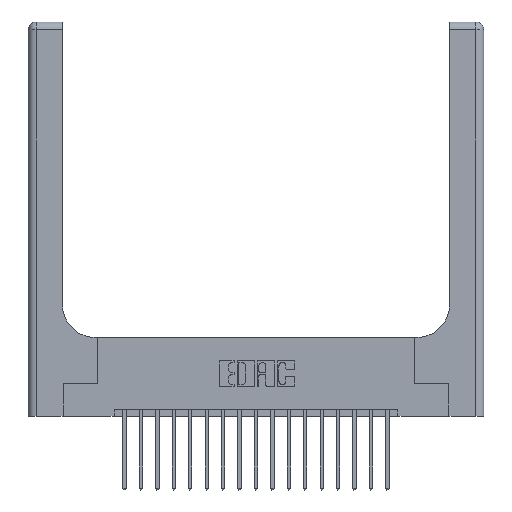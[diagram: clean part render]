
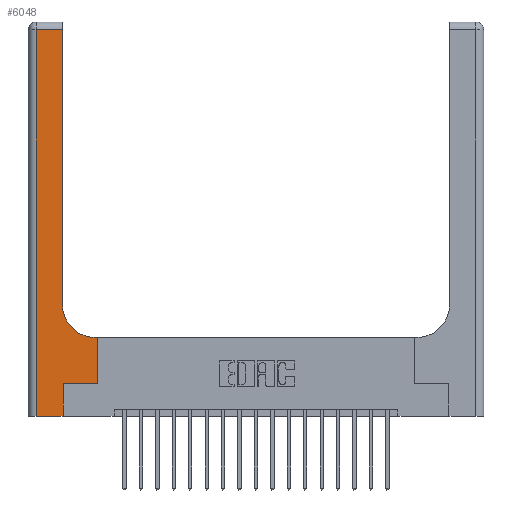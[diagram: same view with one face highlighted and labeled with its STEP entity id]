
A CAD part, top view. The second image highlights one B-rep face of the part: STEP entity #6048.
In plain terms, the highlighted planar face has unit normal (0, 0, 1).
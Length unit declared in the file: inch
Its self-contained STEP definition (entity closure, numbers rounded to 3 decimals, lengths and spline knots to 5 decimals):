
#68 = VERTEX_POINT ( 'NONE', #19939 ) ;
#161 = VERTEX_POINT ( 'NONE', #7725 ) ;
#376 = DIRECTION ( 'NONE',  ( 0., 1., 0. ) ) ;
#683 = CARTESIAN_POINT ( 'NONE',  ( 0.265, 0., 0.37 ) ) ;
#1964 = VERTEX_POINT ( 'NONE', #2599 ) ;
#2024 = CARTESIAN_POINT ( 'NONE',  ( 0.26, 3., 0.37 ) ) ;
#2301 = CARTESIAN_POINT ( 'NONE',  ( 0.26, 0.6, 0.37 ) ) ;
#2599 = CARTESIAN_POINT ( 'NONE',  ( 0.265, 0.25, 0.37 ) ) ;
#2741 = ORIENTED_EDGE ( 'NONE', *, *, #14358, .T. ) ;
#3065 = VECTOR ( 'NONE', #376, 39.37008 ) ;
#3372 = CARTESIAN_POINT ( 'NONE',  ( 0.528, 0.25, 0.37 ) ) ;
#3415 = ORIENTED_EDGE ( 'NONE', *, *, #6404, .T. ) ;
#3646 = VECTOR ( 'NONE', #11444, 39.37008 ) ;
#3700 = DIRECTION ( 'NONE',  ( -1., 0., 0. ) ) ;
#3851 = CARTESIAN_POINT ( 'NONE',  ( 0.06, 3., 0.37 ) ) ;
#3950 = EDGE_CURVE ( 'NONE', #161, #14407, #9134, .T. ) ;
#4714 = EDGE_CURVE ( 'NONE', #15654, #68, #10905, .T. ) ;
#5077 = CARTESIAN_POINT ( 'NONE',  ( 0.528, 0.6, 0.37 ) ) ;
#5481 = ORIENTED_EDGE ( 'NONE', *, *, #16665, .T. ) ;
#5692 = VECTOR ( 'NONE', #7218, 39.37008 ) ;
#5764 = CARTESIAN_POINT ( 'NONE',  ( 0.51, 0.6, 0.37 ) ) ;
#5908 = VECTOR ( 'NONE', #16442, 39.37008 ) ;
#6048 = ADVANCED_FACE ( 'NONE', ( #12311 ), #9370, .F. ) ;
#6404 = EDGE_CURVE ( 'NONE', #18203, #13740, #6736, .T. ) ;
#6592 = LINE ( 'NONE', #2024, #3065 ) ;
#6636 = VERTEX_POINT ( 'NONE', #3372 ) ;
#6736 = LINE ( 'NONE', #12910, #15665 ) ;
#7095 = DIRECTION ( 'NONE',  ( 0., -1., 0. ) ) ;
#7218 = DIRECTION ( 'NONE',  ( 1., 0., 0. ) ) ;
#7239 = ORIENTED_EDGE ( 'NONE', *, *, #19558, .T. ) ;
#7725 = CARTESIAN_POINT ( 'NONE',  ( 0.06, 0., 0.37 ) ) ;
#7795 = EDGE_CURVE ( 'NONE', #10667, #15654, #19387, .T. ) ;
#8059 = AXIS2_PLACEMENT_3D ( 'NONE', #18850, #13858, #12709 ) ;
#8204 = CARTESIAN_POINT ( 'NONE',  ( 0.26, 2.94, 0.37 ) ) ;
#8319 = LINE ( 'NONE', #17468, #3646 ) ;
#8814 = LINE ( 'NONE', #3851, #13497 ) ;
#9134 = LINE ( 'NONE', #19725, #5692 ) ;
#9370 = PLANE ( 'NONE',  #8059 ) ;
#9966 = DIRECTION ( 'NONE',  ( 1., 0., 0. ) ) ;
#10273 = DIRECTION ( 'NONE',  ( 0., 0., -1. ) ) ;
#10667 = VERTEX_POINT ( 'NONE', #5077 ) ;
#10905 = CIRCLE ( 'NONE', #15479, 0.25 ) ;
#11444 = DIRECTION ( 'NONE',  ( 0., 1., 0. ) ) ;
#11721 = VECTOR ( 'NONE', #14621, 39.37008 ) ;
#12311 = FACE_OUTER_BOUND ( 'NONE', #15535, .T. ) ;
#12709 = DIRECTION ( 'NONE',  ( -1., 0., 0. ) ) ;
#12910 = CARTESIAN_POINT ( 'NONE',  ( 0., 2.94, 0.37 ) ) ;
#13008 = ORIENTED_EDGE ( 'NONE', *, *, #3950, .T. ) ;
#13131 = DIRECTION ( 'NONE',  ( -1., 0., 0. ) ) ;
#13302 = CARTESIAN_POINT ( 'NONE',  ( 0.51, 0.85, 0.37 ) ) ;
#13497 = VECTOR ( 'NONE', #7095, 39.37008 ) ;
#13690 = CARTESIAN_POINT ( 'NONE',  ( 0.265, 0.25, 0.37 ) ) ;
#13740 = VERTEX_POINT ( 'NONE', #14294 ) ;
#13858 = DIRECTION ( 'NONE',  ( 0., 0., -1. ) ) ;
#14294 = CARTESIAN_POINT ( 'NONE',  ( 0.06, 2.94, 0.37 ) ) ;
#14358 = EDGE_CURVE ( 'NONE', #14407, #1964, #19202, .T. ) ;
#14363 = EDGE_CURVE ( 'NONE', #6636, #10667, #8319, .T. ) ;
#14407 = VERTEX_POINT ( 'NONE', #17572 ) ;
#14474 = EDGE_CURVE ( 'NONE', #1964, #6636, #18301, .T. ) ;
#14577 = ORIENTED_EDGE ( 'NONE', *, *, #7795, .T. ) ;
#14621 = DIRECTION ( 'NONE',  ( 0., 1., 0. ) ) ;
#15479 = AXIS2_PLACEMENT_3D ( 'NONE', #13302, #10273, #9966 ) ;
#15535 = EDGE_LOOP ( 'NONE', ( #5481, #3415, #7239, #13008, #2741, #19279, #19851, #14577, #17604 ) ) ;
#15654 = VERTEX_POINT ( 'NONE', #5764 ) ;
#15665 = VECTOR ( 'NONE', #3700, 39.37008 ) ;
#16442 = DIRECTION ( 'NONE',  ( 1., 0., 0. ) ) ;
#16665 = EDGE_CURVE ( 'NONE', #68, #18203, #6592, .T. ) ;
#17468 = CARTESIAN_POINT ( 'NONE',  ( 0.528, 0.25, 0.37 ) ) ;
#17572 = CARTESIAN_POINT ( 'NONE',  ( 0.265, 0., 0.37 ) ) ;
#17604 = ORIENTED_EDGE ( 'NONE', *, *, #4714, .T. ) ;
#18203 = VERTEX_POINT ( 'NONE', #8204 ) ;
#18301 = LINE ( 'NONE', #13690, #5908 ) ;
#18850 = CARTESIAN_POINT ( 'NONE',  ( 0., 3., 0.37 ) ) ;
#19070 = VECTOR ( 'NONE', #13131, 39.37008 ) ;
#19202 = LINE ( 'NONE', #683, #11721 ) ;
#19279 = ORIENTED_EDGE ( 'NONE', *, *, #14474, .T. ) ;
#19387 = LINE ( 'NONE', #2301, #19070 ) ;
#19558 = EDGE_CURVE ( 'NONE', #13740, #161, #8814, .T. ) ;
#19725 = CARTESIAN_POINT ( 'NONE',  ( 0., 0., 0.37 ) ) ;
#19851 = ORIENTED_EDGE ( 'NONE', *, *, #14363, .T. ) ;
#19939 = CARTESIAN_POINT ( 'NONE',  ( 0.26, 0.85, 0.37 ) ) ;
